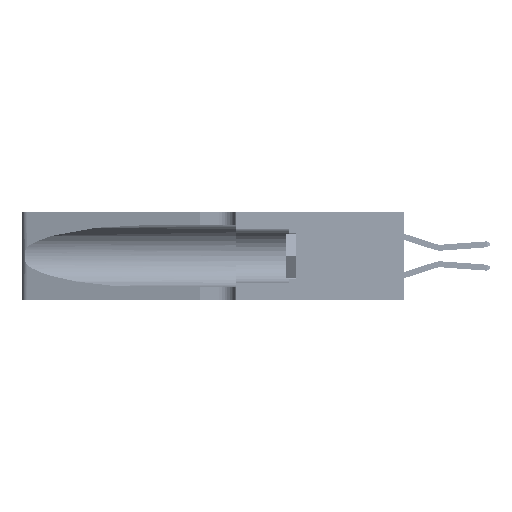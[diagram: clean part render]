
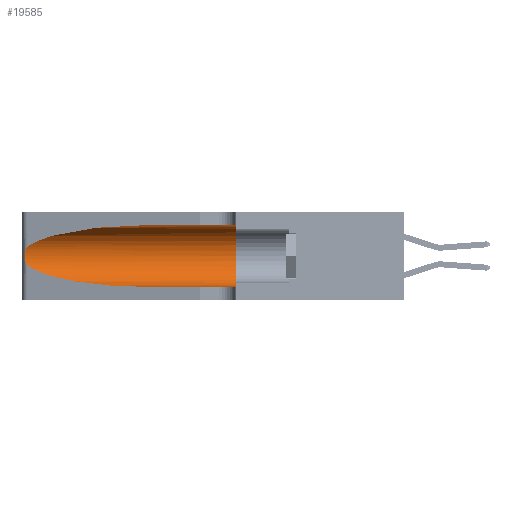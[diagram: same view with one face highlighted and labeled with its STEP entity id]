
A CAD part, left-side view. The second image highlights one B-rep face of the part: STEP entity #19585.
In plain terms, the highlighted cylindrical face has radius 3.308 mm (diameter 6.617 mm), a partial arc.
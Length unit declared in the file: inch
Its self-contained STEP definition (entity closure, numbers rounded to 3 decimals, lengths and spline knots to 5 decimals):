
#214 = CARTESIAN_POINT ( 'NONE',  ( 0.18966, 0.96281, 0.05475 ) ) ;
#354 = LINE ( 'NONE', #28823, #31609 ) ;
#391 = B_SPLINE_CURVE_WITH_KNOTS ( 'NONE', 3,
 ( #34876, #20401, #45806, #24079, #2288, #27710, #5924, #34244, #42466, #6548, #24235, #20539, #46273, #28352 ),
 .UNSPECIFIED., .F., .F.,
 ( 4, 2, 2, 2, 2, 2, 4 ),
 ( 0., 0.00027, 0.00053, 0.00107, 0.0016, 0.00187, 0.00214 ),
 .UNSPECIFIED. ) ;
#409 = ORIENTED_EDGE ( 'NONE', *, *, #18834, .F. ) ;
#2288 = CARTESIAN_POINT ( 'NONE',  ( 0.25854, 1.2359, 0.20912 ) ) ;
#2502 = CARTESIAN_POINT ( 'NONE',  ( 0.1305, 0.72297, 0.31525 ) ) ;
#3162 = CARTESIAN_POINT ( 'NONE',  ( 0.1305, 0.35, 0.31525 ) ) ;
#4018 = CARTESIAN_POINT ( 'NONE',  ( 0.2373, 1.15595, 0.08982 ) ) ;
#5685 = EDGE_CURVE ( 'NONE', #42577, #34913, #31516, .T. ) ;
#5924 = CARTESIAN_POINT ( 'NONE',  ( 0.26075, 1.23896, 0.19203 ) ) ;
#6194 = CIRCLE ( 'NONE', #13403, 0.13025 ) ;
#6548 = CARTESIAN_POINT ( 'NONE',  ( 0.25856, 1.23593, 0.16098 ) ) ;
#7172 = CARTESIAN_POINT ( 'NONE',  ( 0.1305, 0.72297, 0.31525 ) ) ;
#8066 = CARTESIAN_POINT ( 'NONE',  ( 0.25487, 1.22718, 0.22369 ) ) ;
#8127 = EDGE_CURVE ( 'NONE', #33678, #8175, #32133, .T. ) ;
#8175 = VERTEX_POINT ( 'NONE', #25671 ) ;
#8571 = ORIENTED_EDGE ( 'NONE', *, *, #8127, .T. ) ;
#9174 = CARTESIAN_POINT ( 'NONE',  ( 0.1305, 1.61858, 0.05475 ) ) ;
#13339 = EDGE_CURVE ( 'NONE', #8175, #27196, #24790, .T. ) ;
#13403 = AXIS2_PLACEMENT_3D ( 'NONE', #26834, #34135, #23179 ) ;
#16432 = DIRECTION ( 'NONE',  ( 0., -1., 0. ) ) ;
#17664 = ORIENTED_EDGE ( 'NONE', *, *, #5685, .T. ) ;
#18812 = CARTESIAN_POINT ( 'NONE',  ( 0.25487, 1.22718, 0.14631 ) ) ;
#18834 = EDGE_CURVE ( 'NONE', #42577, #20461, #354, .T. ) ;
#19585 = ADVANCED_FACE ( 'NONE', ( #23636 ), #21310, .F. ) ;
#20067 = DIRECTION ( 'NONE',  ( 0., 0., -1. ) ) ;
#20401 = CARTESIAN_POINT ( 'NONE',  ( 0.25555, 1.22994, 0.2215 ) ) ;
#20461 = VERTEX_POINT ( 'NONE', #3162 ) ;
#20539 = CARTESIAN_POINT ( 'NONE',  ( 0.25639, 1.23186, 0.15144 ) ) ;
#20906 = AXIS2_PLACEMENT_3D ( 'NONE', #38201, #16432, #20067 ) ;
#21310 = CYLINDRICAL_SURFACE ( 'NONE', #20906, 0.13025 ) ;
#22960 = EDGE_CURVE ( 'NONE', #20461, #27196, #6194, .T. ) ;
#23179 = DIRECTION ( 'NONE',  ( 0., 0., 1. ) ) ;
#23636 = FACE_OUTER_BOUND ( 'NONE', #34513, .T. ) ;
#24079 = CARTESIAN_POINT ( 'NONE',  ( 0.25787, 1.23484, 0.2124 ) ) ;
#24161 = CARTESIAN_POINT ( 'NONE',  ( 0.2373, 1.15595, 0.28018 ) ) ;
#24235 = CARTESIAN_POINT ( 'NONE',  ( 0.25789, 1.23486, 0.15765 ) ) ;
#24790 = LINE ( 'NONE', #9174, #29887 ) ;
#24990 = ORIENTED_EDGE ( 'NONE', *, *, #22960, .F. ) ;
#25671 = CARTESIAN_POINT ( 'NONE',  ( 0.1305, 0.72297, 0.05475 ) ) ;
#26834 = CARTESIAN_POINT ( 'NONE',  ( 0.1305, 0.35, 0.185 ) ) ;
#27196 = VERTEX_POINT ( 'NONE', #44644 ) ;
#27710 = CARTESIAN_POINT ( 'NONE',  ( 0.26018, 1.23835, 0.19895 ) ) ;
#28352 = CARTESIAN_POINT ( 'NONE',  ( 0.25487, 1.22718, 0.14631 ) ) ;
#28823 = CARTESIAN_POINT ( 'NONE',  ( 0.1305, 1.61858, 0.31525 ) ) ;
#29690 = EDGE_CURVE ( 'NONE', #34913, #33678, #391, .T. ) ;
#29887 = VECTOR ( 'NONE', #31709, 39.37008 ) ;
#31516 =( BOUNDED_CURVE ( )  B_SPLINE_CURVE ( 3, ( #2502, #38438, #24161, #34657 ),
 .UNSPECIFIED., .F., .F. ) 
 B_SPLINE_CURVE_WITH_KNOTS ( ( 4, 4 ),
 ( 1.5708, 2.84003 ),
 .UNSPECIFIED. ) 
 CURVE ( )  GEOMETRIC_REPRESENTATION_ITEM ( )  RATIONAL_B_SPLINE_CURVE ( ( 1., 0.87, 0.87, 1. ) ) 
 REPRESENTATION_ITEM ( '' )  );
#31609 = VECTOR ( 'NONE', #32483, 39.37008 ) ;
#31709 = DIRECTION ( 'NONE',  ( 0., -1., 0. ) ) ;
#32133 =( BOUNDED_CURVE ( )  B_SPLINE_CURVE ( 3, ( #18812, #4018, #214, #43742 ),
 .UNSPECIFIED., .F., .T. ) 
 B_SPLINE_CURVE_WITH_KNOTS ( ( 4, 4 ),
 ( 3.44316, 4.71239 ),
 .UNSPECIFIED. ) 
 CURVE ( )  GEOMETRIC_REPRESENTATION_ITEM ( )  RATIONAL_B_SPLINE_CURVE ( ( 1., 0.87, 0.87, 1. ) ) 
 REPRESENTATION_ITEM ( '' )  );
#32483 = DIRECTION ( 'NONE',  ( 0., -1., 0. ) ) ;
#33297 = ORIENTED_EDGE ( 'NONE', *, *, #29690, .T. ) ;
#33678 = VERTEX_POINT ( 'NONE', #38982 ) ;
#34135 = DIRECTION ( 'NONE',  ( 0., 1., 0. ) ) ;
#34150 = ORIENTED_EDGE ( 'NONE', *, *, #13339, .T. ) ;
#34244 = CARTESIAN_POINT ( 'NONE',  ( 0.26075, 1.23896, 0.178 ) ) ;
#34513 = EDGE_LOOP ( 'NONE', ( #17664, #33297, #8571, #34150, #24990, #409 ) ) ;
#34657 = CARTESIAN_POINT ( 'NONE',  ( 0.25487, 1.22718, 0.22369 ) ) ;
#34876 = CARTESIAN_POINT ( 'NONE',  ( 0.25487, 1.22718, 0.22369 ) ) ;
#34913 = VERTEX_POINT ( 'NONE', #8066 ) ;
#38201 = CARTESIAN_POINT ( 'NONE',  ( 0.1305, 1.61858, 0.185 ) ) ;
#38438 = CARTESIAN_POINT ( 'NONE',  ( 0.18966, 0.96281, 0.31525 ) ) ;
#38982 = CARTESIAN_POINT ( 'NONE',  ( 0.25487, 1.22718, 0.14631 ) ) ;
#42466 = CARTESIAN_POINT ( 'NONE',  ( 0.26017, 1.23833, 0.17102 ) ) ;
#42577 = VERTEX_POINT ( 'NONE', #7172 ) ;
#43742 = CARTESIAN_POINT ( 'NONE',  ( 0.1305, 0.72297, 0.05475 ) ) ;
#44644 = CARTESIAN_POINT ( 'NONE',  ( 0.1305, 0.35, 0.05475 ) ) ;
#45806 = CARTESIAN_POINT ( 'NONE',  ( 0.25639, 1.23184, 0.21858 ) ) ;
#46273 = CARTESIAN_POINT ( 'NONE',  ( 0.25555, 1.22993, 0.14849 ) ) ;
